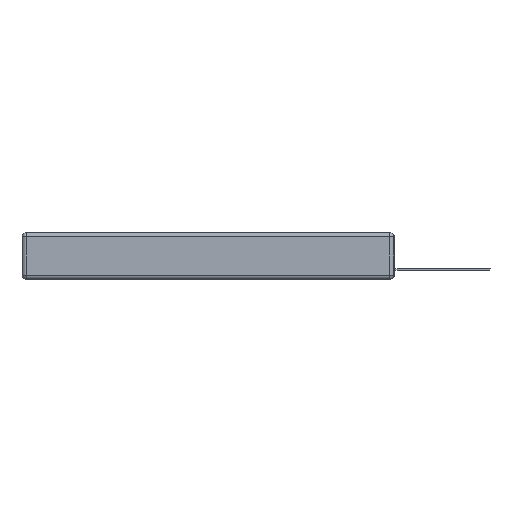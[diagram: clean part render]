
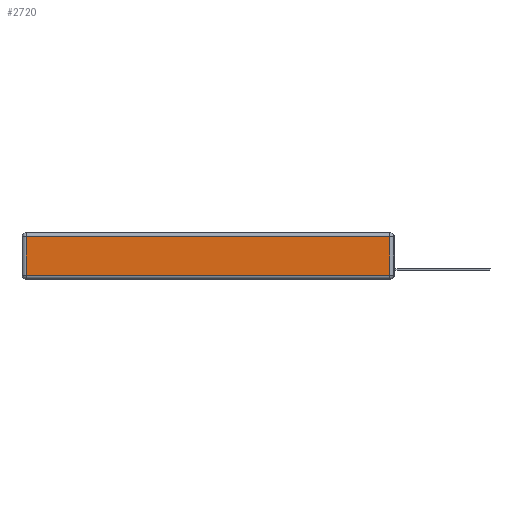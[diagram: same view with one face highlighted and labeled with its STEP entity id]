
A CAD part, left-side view. The second image highlights one B-rep face of the part: STEP entity #2720.
In plain terms, the highlighted planar face has unit normal (-1, 0, 0).
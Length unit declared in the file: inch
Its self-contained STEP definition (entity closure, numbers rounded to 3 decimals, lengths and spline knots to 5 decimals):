
#161 = ORIENTED_EDGE ( 'NONE', *, *, #5667, .T. ) ;
#162 = CARTESIAN_POINT ( 'NONE',  ( 0., 0.03, -0.03 ) ) ;
#271 = PLANE ( 'NONE',  #2998 ) ;
#619 = FACE_OUTER_BOUND ( 'NONE', #7035, .T. ) ;
#1017 = LINE ( 'NONE', #4343, #4847 ) ;
#1221 = DIRECTION ( 'NONE',  ( -1., 0., 0. ) ) ;
#1582 = CARTESIAN_POINT ( 'NONE',  ( 0., 0.03, -0.313 ) ) ;
#1737 = VERTEX_POINT ( 'NONE', #1582 ) ;
#2088 = VERTEX_POINT ( 'NONE', #11029 ) ;
#2720 = ADVANCED_FACE ( 'NONE', ( #619 ), #271, .T. ) ;
#2954 = CARTESIAN_POINT ( 'NONE',  ( 0., 0., -0.343 ) ) ;
#2998 = AXIS2_PLACEMENT_3D ( 'NONE', #2954, #1221, #6873 ) ;
#3377 = LINE ( 'NONE', #3973, #8007 ) ;
#3590 = DIRECTION ( 'NONE',  ( 0., 0., 1. ) ) ;
#3973 = CARTESIAN_POINT ( 'NONE',  ( 0., 2.72, -0.343 ) ) ;
#4174 = DIRECTION ( 'NONE',  ( 0., -1., 0. ) ) ;
#4343 = CARTESIAN_POINT ( 'NONE',  ( 0., 2.75, -0.03 ) ) ;
#4462 = CARTESIAN_POINT ( 'NONE',  ( 0., 0.03, -0.343 ) ) ;
#4782 = LINE ( 'NONE', #4462, #9255 ) ;
#4847 = VECTOR ( 'NONE', #11730, 39.37008 ) ;
#4950 = DIRECTION ( 'NONE',  ( 0., 0., -1. ) ) ;
#5070 = VERTEX_POINT ( 'NONE', #162 ) ;
#5148 = EDGE_CURVE ( 'NONE', #5919, #2088, #3377, .T. ) ;
#5217 = EDGE_CURVE ( 'NONE', #5070, #5919, #1017, .T. ) ;
#5313 = CARTESIAN_POINT ( 'NONE',  ( 0., 2.72, -0.03 ) ) ;
#5667 = EDGE_CURVE ( 'NONE', #2088, #1737, #8442, .T. ) ;
#5919 = VERTEX_POINT ( 'NONE', #5313 ) ;
#5965 = CARTESIAN_POINT ( 'NONE',  ( 0., 0., -0.313 ) ) ;
#6628 = ORIENTED_EDGE ( 'NONE', *, *, #7844, .T. ) ;
#6873 = DIRECTION ( 'NONE',  ( 0., 0., 1. ) ) ;
#7035 = EDGE_LOOP ( 'NONE', ( #161, #6628, #8654, #8804 ) ) ;
#7517 = VECTOR ( 'NONE', #4174, 39.37008 ) ;
#7844 = EDGE_CURVE ( 'NONE', #1737, #5070, #4782, .T. ) ;
#8007 = VECTOR ( 'NONE', #4950, 39.37008 ) ;
#8442 = LINE ( 'NONE', #5965, #7517 ) ;
#8654 = ORIENTED_EDGE ( 'NONE', *, *, #5217, .T. ) ;
#8804 = ORIENTED_EDGE ( 'NONE', *, *, #5148, .T. ) ;
#9255 = VECTOR ( 'NONE', #3590, 39.37008 ) ;
#11029 = CARTESIAN_POINT ( 'NONE',  ( 0., 2.72, -0.313 ) ) ;
#11730 = DIRECTION ( 'NONE',  ( 0., 1., 0. ) ) ;
